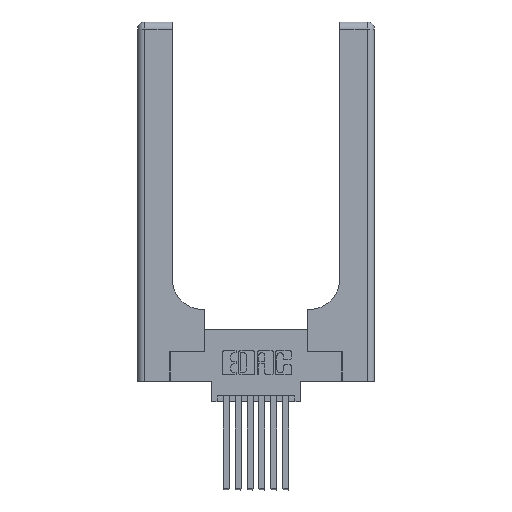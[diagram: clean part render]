
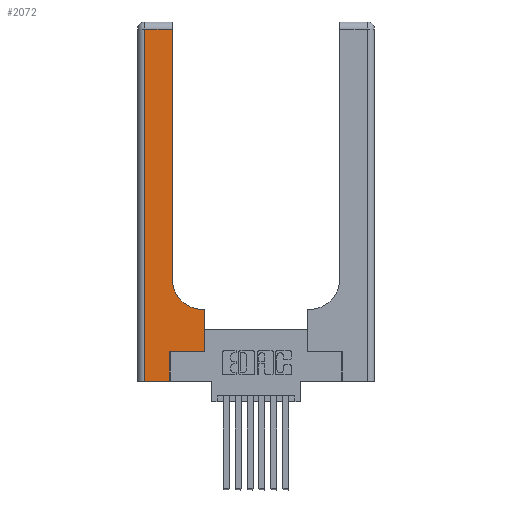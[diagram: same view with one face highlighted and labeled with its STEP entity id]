
A CAD part, top view. The second image highlights one B-rep face of the part: STEP entity #2072.
In plain terms, the highlighted planar face has unit normal (0, 0, 1).
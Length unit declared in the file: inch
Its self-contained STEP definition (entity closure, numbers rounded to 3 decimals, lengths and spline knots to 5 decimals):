
#161 = DIRECTION ( 'NONE',  ( 0., -1., 0. ) ) ;
#305 = CARTESIAN_POINT ( 'NONE',  ( 0.5585, 0.25, 0.37 ) ) ;
#512 = VECTOR ( 'NONE', #4563, 39.37008 ) ;
#588 = LINE ( 'NONE', #305, #3333 ) ;
#674 = EDGE_CURVE ( 'NONE', #3902, #10824, #12136, .T. ) ;
#721 = EDGE_CURVE ( 'NONE', #4819, #3764, #8786, .T. ) ;
#730 = DIRECTION ( 'NONE',  ( 0., 0., -1. ) ) ;
#827 = LINE ( 'NONE', #6064, #1194 ) ;
#1133 = ORIENTED_EDGE ( 'NONE', *, *, #11736, .T. ) ;
#1194 = VECTOR ( 'NONE', #13928, 39.37008 ) ;
#1347 = CARTESIAN_POINT ( 'NONE',  ( 0.06, 3., 0.37 ) ) ;
#1388 = VERTEX_POINT ( 'NONE', #6203 ) ;
#1852 = LINE ( 'NONE', #2220, #4519 ) ;
#1912 = CARTESIAN_POINT ( 'NONE',  ( 0.269, 0., 0.37 ) ) ;
#2072 = ADVANCED_FACE ( 'NONE', ( #9139 ), #8695, .F. ) ;
#2220 = CARTESIAN_POINT ( 'NONE',  ( 0., 0., 0.37 ) ) ;
#2259 = CARTESIAN_POINT ( 'NONE',  ( 0.269, 0.25, 0.37 ) ) ;
#2275 = VERTEX_POINT ( 'NONE', #10719 ) ;
#2823 = EDGE_CURVE ( 'NONE', #3764, #3902, #588, .T. ) ;
#3333 = VECTOR ( 'NONE', #10512, 39.37008 ) ;
#3378 = DIRECTION ( 'NONE',  ( 1., 0., 0. ) ) ;
#3683 = ORIENTED_EDGE ( 'NONE', *, *, #4060, .T. ) ;
#3764 = VERTEX_POINT ( 'NONE', #5533 ) ;
#3902 = VERTEX_POINT ( 'NONE', #5880 ) ;
#4060 = EDGE_CURVE ( 'NONE', #10824, #7742, #6635, .T. ) ;
#4204 = ORIENTED_EDGE ( 'NONE', *, *, #7384, .T. ) ;
#4213 = EDGE_CURVE ( 'NONE', #1388, #2275, #1852, .T. ) ;
#4519 = VECTOR ( 'NONE', #3378, 39.37008 ) ;
#4555 = ORIENTED_EDGE ( 'NONE', *, *, #7302, .T. ) ;
#4563 = DIRECTION ( 'NONE',  ( 0., 1., 0. ) ) ;
#4819 = VERTEX_POINT ( 'NONE', #2259 ) ;
#5021 = CARTESIAN_POINT ( 'NONE',  ( 0.5415, 0.6, 0.37 ) ) ;
#5204 = CARTESIAN_POINT ( 'NONE',  ( 0.2915, 2.94, 0.37 ) ) ;
#5246 = ORIENTED_EDGE ( 'NONE', *, *, #721, .T. ) ;
#5533 = CARTESIAN_POINT ( 'NONE',  ( 0.5585, 0.25, 0.37 ) ) ;
#5611 = VECTOR ( 'NONE', #9764, 39.37008 ) ;
#5723 = VERTEX_POINT ( 'NONE', #7054 ) ;
#5818 = EDGE_LOOP ( 'NONE', ( #1133, #4204, #4555, #10848, #13876, #5246, #8209, #8574, #3683 ) ) ;
#5880 = CARTESIAN_POINT ( 'NONE',  ( 0.5585, 0.6, 0.37 ) ) ;
#6064 = CARTESIAN_POINT ( 'NONE',  ( 0., 2.94, 0.37 ) ) ;
#6171 = VECTOR ( 'NONE', #12603, 39.37008 ) ;
#6203 = CARTESIAN_POINT ( 'NONE',  ( 0.06, 0., 0.37 ) ) ;
#6635 = CIRCLE ( 'NONE', #8188, 0.25 ) ;
#7054 = CARTESIAN_POINT ( 'NONE',  ( 0.06, 2.94, 0.37 ) ) ;
#7302 = EDGE_CURVE ( 'NONE', #5723, #1388, #13585, .T. ) ;
#7384 = EDGE_CURVE ( 'NONE', #12802, #5723, #827, .T. ) ;
#7512 = CARTESIAN_POINT ( 'NONE',  ( 0.5415, 0.85, 0.37 ) ) ;
#7742 = VERTEX_POINT ( 'NONE', #11297 ) ;
#8188 = AXIS2_PLACEMENT_3D ( 'NONE', #7512, #730, #8658 ) ;
#8209 = ORIENTED_EDGE ( 'NONE', *, *, #2823, .T. ) ;
#8371 = AXIS2_PLACEMENT_3D ( 'NONE', #8694, #11025, #11519 ) ;
#8574 = ORIENTED_EDGE ( 'NONE', *, *, #674, .T. ) ;
#8584 = LINE ( 'NONE', #1912, #5611 ) ;
#8658 = DIRECTION ( 'NONE',  ( 1., 0., 0. ) ) ;
#8694 = CARTESIAN_POINT ( 'NONE',  ( 0., 3., 0.37 ) ) ;
#8695 = PLANE ( 'NONE',  #8371 ) ;
#8730 = EDGE_CURVE ( 'NONE', #2275, #4819, #8584, .T. ) ;
#8786 = LINE ( 'NONE', #12329, #14425 ) ;
#9139 = FACE_OUTER_BOUND ( 'NONE', #5818, .T. ) ;
#9555 = LINE ( 'NONE', #13562, #512 ) ;
#9764 = DIRECTION ( 'NONE',  ( 0., 1., 0. ) ) ;
#10512 = DIRECTION ( 'NONE',  ( 0., 1., 0. ) ) ;
#10719 = CARTESIAN_POINT ( 'NONE',  ( 0.269, 0., 0.37 ) ) ;
#10824 = VERTEX_POINT ( 'NONE', #5021 ) ;
#10848 = ORIENTED_EDGE ( 'NONE', *, *, #4213, .T. ) ;
#11025 = DIRECTION ( 'NONE',  ( 0., 0., -1. ) ) ;
#11297 = CARTESIAN_POINT ( 'NONE',  ( 0.2915, 0.85, 0.37 ) ) ;
#11519 = DIRECTION ( 'NONE',  ( -1., 0., 0. ) ) ;
#11736 = EDGE_CURVE ( 'NONE', #7742, #12802, #9555, .T. ) ;
#12136 = LINE ( 'NONE', #12748, #6171 ) ;
#12299 = DIRECTION ( 'NONE',  ( 1., 0., 0. ) ) ;
#12329 = CARTESIAN_POINT ( 'NONE',  ( 0.269, 0.25, 0.37 ) ) ;
#12603 = DIRECTION ( 'NONE',  ( -1., 0., 0. ) ) ;
#12748 = CARTESIAN_POINT ( 'NONE',  ( 0.2915, 0.6, 0.37 ) ) ;
#12802 = VERTEX_POINT ( 'NONE', #5204 ) ;
#13562 = CARTESIAN_POINT ( 'NONE',  ( 0.2915, 3., 0.37 ) ) ;
#13585 = LINE ( 'NONE', #1347, #13925 ) ;
#13876 = ORIENTED_EDGE ( 'NONE', *, *, #8730, .T. ) ;
#13925 = VECTOR ( 'NONE', #161, 39.37008 ) ;
#13928 = DIRECTION ( 'NONE',  ( -1., 0., 0. ) ) ;
#14425 = VECTOR ( 'NONE', #12299, 39.37008 ) ;
